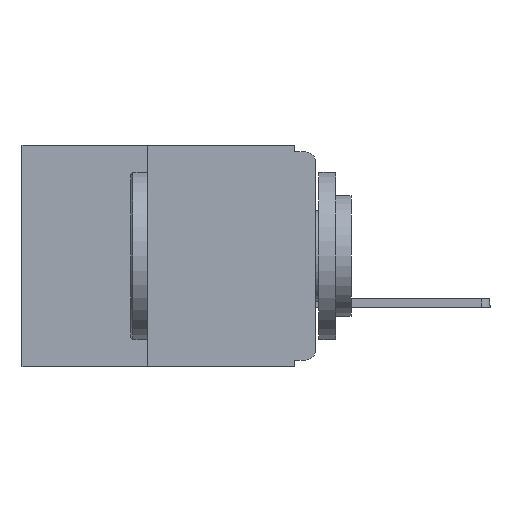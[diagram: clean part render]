
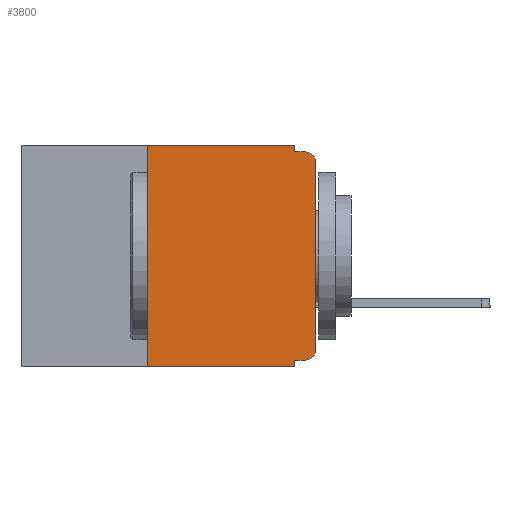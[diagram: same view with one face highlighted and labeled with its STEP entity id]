
A CAD part, left-side view. The second image highlights one B-rep face of the part: STEP entity #3800.
In plain terms, the highlighted planar face has unit normal (-1, 0, 0).
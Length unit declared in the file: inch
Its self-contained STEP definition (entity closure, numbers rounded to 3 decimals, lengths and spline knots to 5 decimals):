
#16 = VERTEX_POINT ( 'NONE', #19690 ) ;
#146 = ORIENTED_EDGE ( 'NONE', *, *, #2476, .F. ) ;
#278 = CARTESIAN_POINT ( 'NONE',  ( 0., 0.25, -0.33 ) ) ;
#1268 = CARTESIAN_POINT ( 'NONE',  ( 0., 0.015, -0.32 ) ) ;
#1408 = CARTESIAN_POINT ( 'NONE',  ( 0., 0.25, -0.33 ) ) ;
#1816 = CARTESIAN_POINT ( 'NONE',  ( 0., 0.031, -0.33 ) ) ;
#2172 = CARTESIAN_POINT ( 'NONE',  ( 0., 0.031, -0.33 ) ) ;
#2476 = EDGE_CURVE ( 'NONE', #9346, #18205, #3630, .T. ) ;
#2843 = EDGE_CURVE ( 'NONE', #16398, #4972, #8845, .T. ) ;
#3023 = CARTESIAN_POINT ( 'NONE',  ( 0., 0.015, -0.025 ) ) ;
#3047 = VECTOR ( 'NONE', #10882, 39.37008 ) ;
#3563 = VERTEX_POINT ( 'NONE', #1268 ) ;
#3630 = LINE ( 'NONE', #1816, #3047 ) ;
#3800 = ADVANCED_FACE ( 'NONE', ( #11806 ), #17557, .F. ) ;
#3817 = ORIENTED_EDGE ( 'NONE', *, *, #6319, .F. ) ;
#4798 = DIRECTION ( 'NONE',  ( 0., 0., -1. ) ) ;
#4905 = ORIENTED_EDGE ( 'NONE', *, *, #12784, .F. ) ;
#4972 = VERTEX_POINT ( 'NONE', #15897 ) ;
#5343 = AXIS2_PLACEMENT_3D ( 'NONE', #16047, #5719, #17763 ) ;
#5719 = DIRECTION ( 'NONE',  ( -1., 0., 0. ) ) ;
#6035 = DIRECTION ( 'NONE',  ( 0., 0., 1. ) ) ;
#6234 = CARTESIAN_POINT ( 'NONE',  ( 0., 0., -0.01 ) ) ;
#6319 = EDGE_CURVE ( 'NONE', #4972, #16, #10061, .T. ) ;
#6619 = CARTESIAN_POINT ( 'NONE',  ( 0., 0.015, -0.01 ) ) ;
#6828 = ORIENTED_EDGE ( 'NONE', *, *, #11449, .T. ) ;
#6973 = CARTESIAN_POINT ( 'NONE',  ( 0., 0.437, 0. ) ) ;
#6981 = CARTESIAN_POINT ( 'NONE',  ( 0., 0.031, -0.32 ) ) ;
#6996 = CARTESIAN_POINT ( 'NONE',  ( 0., 0.437, 0. ) ) ;
#7168 = VECTOR ( 'NONE', #21213, 39.37008 ) ;
#7665 = VERTEX_POINT ( 'NONE', #14019 ) ;
#7769 = EDGE_CURVE ( 'NONE', #3563, #19409, #10031, .T. ) ;
#7869 = EDGE_CURVE ( 'NONE', #19409, #17463, #8361, .T. ) ;
#8361 = LINE ( 'NONE', #11367, #12429 ) ;
#8506 = ORIENTED_EDGE ( 'NONE', *, *, #2843, .F. ) ;
#8845 = LINE ( 'NONE', #1408, #17364 ) ;
#8952 = VECTOR ( 'NONE', #20628, 39.37008 ) ;
#8953 = CARTESIAN_POINT ( 'NONE',  ( 0., 0., -0.025 ) ) ;
#9164 = CARTESIAN_POINT ( 'NONE',  ( 0., 0.437, -0.33 ) ) ;
#9346 = VERTEX_POINT ( 'NONE', #6981 ) ;
#10031 = CIRCLE ( 'NONE', #5343, 0.015 ) ;
#10061 = LINE ( 'NONE', #6973, #8952 ) ;
#10173 = ORIENTED_EDGE ( 'NONE', *, *, #7769, .T. ) ;
#10882 = DIRECTION ( 'NONE',  ( 0., 0., -1. ) ) ;
#10942 = DIRECTION ( 'NONE',  ( 0., -1., 0. ) ) ;
#11025 = VECTOR ( 'NONE', #11808, 39.37008 ) ;
#11367 = CARTESIAN_POINT ( 'NONE',  ( 0., 0., 0. ) ) ;
#11449 = EDGE_CURVE ( 'NONE', #17463, #15466, #16863, .T. ) ;
#11806 = FACE_OUTER_BOUND ( 'NONE', #19293, .T. ) ;
#11808 = DIRECTION ( 'NONE',  ( 0., 0., -1. ) ) ;
#11829 = LINE ( 'NONE', #19527, #7168 ) ;
#12038 = ORIENTED_EDGE ( 'NONE', *, *, #18992, .F. ) ;
#12429 = VECTOR ( 'NONE', #6035, 39.37008 ) ;
#12784 = EDGE_CURVE ( 'NONE', #3563, #9346, #11829, .T. ) ;
#13021 = EDGE_CURVE ( 'NONE', #16, #7665, #16003, .T. ) ;
#14019 = CARTESIAN_POINT ( 'NONE',  ( 0., 0.031, -0.01 ) ) ;
#14193 = CARTESIAN_POINT ( 'NONE',  ( 0., 0., -0.305 ) ) ;
#14606 = VECTOR ( 'NONE', #10942, 39.37008 ) ;
#15165 = DIRECTION ( 'NONE',  ( -1., 0., 0. ) ) ;
#15466 = VERTEX_POINT ( 'NONE', #6619 ) ;
#15897 = CARTESIAN_POINT ( 'NONE',  ( 0., 0.25, 0. ) ) ;
#16003 = LINE ( 'NONE', #18496, #11025 ) ;
#16047 = CARTESIAN_POINT ( 'NONE',  ( 0., 0.015, -0.305 ) ) ;
#16398 = VERTEX_POINT ( 'NONE', #278 ) ;
#16863 = CIRCLE ( 'NONE', #17386, 0.015 ) ;
#17259 = DIRECTION ( 'NONE',  ( 0., 0., -1. ) ) ;
#17364 = VECTOR ( 'NONE', #21450, 39.37008 ) ;
#17386 = AXIS2_PLACEMENT_3D ( 'NONE', #3023, #15165, #4798 ) ;
#17463 = VERTEX_POINT ( 'NONE', #8953 ) ;
#17466 = DIRECTION ( 'NONE',  ( 1., 0., 0. ) ) ;
#17557 = PLANE ( 'NONE',  #21904 ) ;
#17573 = ORIENTED_EDGE ( 'NONE', *, *, #21901, .T. ) ;
#17763 = DIRECTION ( 'NONE',  ( 0., 0., -1. ) ) ;
#18120 = VECTOR ( 'NONE', #18248, 39.37008 ) ;
#18205 = VERTEX_POINT ( 'NONE', #2172 ) ;
#18248 = DIRECTION ( 'NONE',  ( 0., -1., 0. ) ) ;
#18496 = CARTESIAN_POINT ( 'NONE',  ( 0., 0.031, 0. ) ) ;
#18992 = EDGE_CURVE ( 'NONE', #7665, #15466, #22009, .T. ) ;
#19293 = EDGE_LOOP ( 'NONE', ( #19934, #6828, #12038, #20983, #3817, #8506, #17573, #146, #4905, #10173 ) ) ;
#19409 = VERTEX_POINT ( 'NONE', #14193 ) ;
#19527 = CARTESIAN_POINT ( 'NONE',  ( 0., 0., -0.32 ) ) ;
#19690 = CARTESIAN_POINT ( 'NONE',  ( 0., 0.031, 0. ) ) ;
#19934 = ORIENTED_EDGE ( 'NONE', *, *, #7869, .T. ) ;
#20116 = LINE ( 'NONE', #9164, #14606 ) ;
#20628 = DIRECTION ( 'NONE',  ( 0., -1., 0. ) ) ;
#20983 = ORIENTED_EDGE ( 'NONE', *, *, #13021, .F. ) ;
#21213 = DIRECTION ( 'NONE',  ( 0., 1., 0. ) ) ;
#21450 = DIRECTION ( 'NONE',  ( 0., 0., 1. ) ) ;
#21901 = EDGE_CURVE ( 'NONE', #16398, #18205, #20116, .T. ) ;
#21904 = AXIS2_PLACEMENT_3D ( 'NONE', #6996, #17466, #17259 ) ;
#22009 = LINE ( 'NONE', #6234, #18120 ) ;
